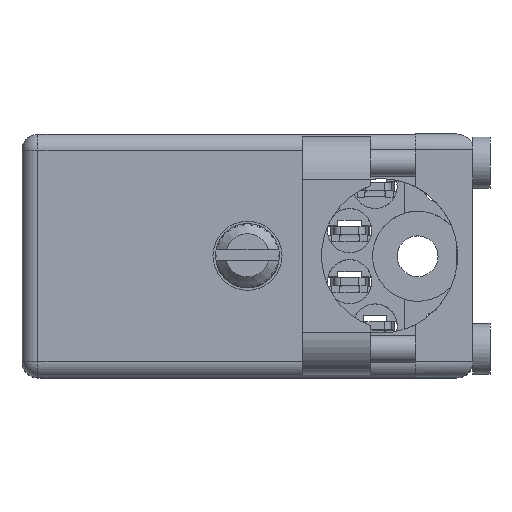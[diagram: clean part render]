
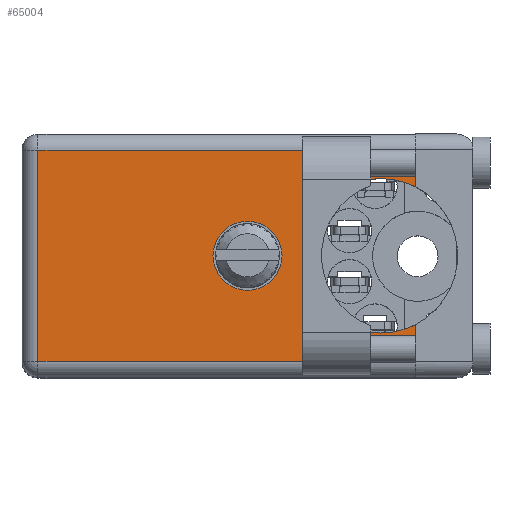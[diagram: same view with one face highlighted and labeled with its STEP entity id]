
A CAD part, top view. The second image highlights one B-rep face of the part: STEP entity #65004.
In plain terms, the highlighted face is planar.
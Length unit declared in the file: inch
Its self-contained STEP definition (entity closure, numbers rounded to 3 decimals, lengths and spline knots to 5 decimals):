
#6867 = AXIS2_PLACEMENT_3D ( 'NONE', #28038, #45267, #128911 ) ;
#7280 = DIRECTION ( 'NONE',  ( -1., 0., 0. ) ) ;
#7720 = CARTESIAN_POINT ( 'NONE',  ( 0.4925, 0.806, -0.3105 ) ) ;
#9717 = EDGE_CURVE ( 'NONE', #14492, #12647, #14792, .T. ) ;
#12647 = VERTEX_POINT ( 'NONE', #168952 ) ;
#12778 = DIRECTION ( 'NONE',  ( 0., 1., 0. ) ) ;
#13889 = AXIS2_PLACEMENT_3D ( 'NONE', #64931, #95680, #7280 ) ;
#14492 = VERTEX_POINT ( 'NONE', #45235 ) ;
#14792 = LINE ( 'NONE', #87786, #27591 ) ;
#18114 = AXIS2_PLACEMENT_3D ( 'NONE', #37521, #50966, #156558 ) ;
#19705 = EDGE_CURVE ( 'NONE', #43490, #105128, #61039, .T. ) ;
#24558 = CIRCLE ( 'NONE', #131970, 0.227 ) ;
#24832 = VERTEX_POINT ( 'NONE', #26908 ) ;
#25369 = ORIENTED_EDGE ( 'NONE', *, *, #111551, .F. ) ;
#26908 = CARTESIAN_POINT ( 'NONE',  ( 0.3905, 0.806, -0.227 ) ) ;
#27200 = CARTESIAN_POINT ( 'NONE',  ( -0.6625, 0.806, -0.3575 ) ) ;
#27327 = CIRCLE ( 'NONE', #18114, 0.227 ) ;
#27591 = VECTOR ( 'NONE', #150162, 39.37008 ) ;
#27747 = LINE ( 'NONE', #142064, #36396 ) ;
#28038 = CARTESIAN_POINT ( 'NONE',  ( 0., 0.806, 0. ) ) ;
#28193 = DIRECTION ( 'NONE',  ( 0., 1., 0. ) ) ;
#31834 = ORIENTED_EDGE ( 'NONE', *, *, #9717, .T. ) ;
#36396 = VECTOR ( 'NONE', #128610, 39.37008 ) ;
#37521 = CARTESIAN_POINT ( 'NONE',  ( 0.3905, 0.806, 0. ) ) ;
#37911 = DIRECTION ( 'NONE',  ( 0., 1., 0. ) ) ;
#40809 = EDGE_CURVE ( 'NONE', #123124, #163807, #27747, .T. ) ;
#41180 = DIRECTION ( 'NONE',  ( 0., 0., 1. ) ) ;
#41448 = CIRCLE ( 'NONE', #13889, 0.227 ) ;
#41816 = ORIENTED_EDGE ( 'NONE', *, *, #19705, .F. ) ;
#43490 = VERTEX_POINT ( 'NONE', #174064 ) ;
#45235 = CARTESIAN_POINT ( 'NONE',  ( -0.6155, 0.806, -0.3105 ) ) ;
#45267 = DIRECTION ( 'NONE',  ( 0., 1., 0. ) ) ;
#46036 = VERTEX_POINT ( 'NONE', #116571 ) ;
#47566 = VERTEX_POINT ( 'NONE', #48930 ) ;
#48930 = CARTESIAN_POINT ( 'NONE',  ( 0.3905, 0.806, 0.227 ) ) ;
#50966 = DIRECTION ( 'NONE',  ( 0., 1., 0. ) ) ;
#52404 = CARTESIAN_POINT ( 'NONE',  ( 0.4925, 0.806, 0.20279 ) ) ;
#59779 = FACE_OUTER_BOUND ( 'NONE', #139218, .T. ) ;
#61039 = CIRCLE ( 'NONE', #6867, 0.1015 ) ;
#64931 = CARTESIAN_POINT ( 'NONE',  ( 0.3905, 0.806, 0. ) ) ;
#65004 = ADVANCED_FACE ( 'NONE', ( #59779, #100188 ), #158760, .T. ) ;
#68299 = EDGE_CURVE ( 'NONE', #24832, #47566, #41448, .T. ) ;
#71351 = DIRECTION ( 'NONE',  ( -1., 0., 0. ) ) ;
#71396 = DIRECTION ( 'NONE',  ( -1., 0., 0. ) ) ;
#74703 = ORIENTED_EDGE ( 'NONE', *, *, #175465, .F. ) ;
#77103 = AXIS2_PLACEMENT_3D ( 'NONE', #27200, #12778, #71351 ) ;
#80381 = CARTESIAN_POINT ( 'NONE',  ( 0.3905, 0.806, 0. ) ) ;
#80827 = LINE ( 'NONE', #123148, #127807 ) ;
#86930 = ORIENTED_EDGE ( 'NONE', *, *, #150568, .T. ) ;
#87745 = AXIS2_PLACEMENT_3D ( 'NONE', #142544, #37911, #100282 ) ;
#87786 = CARTESIAN_POINT ( 'NONE',  ( -0.6155, 0.806, -0.3575 ) ) ;
#89505 = VECTOR ( 'NONE', #162537, 39.37008 ) ;
#90490 = LINE ( 'NONE', #123118, #89505 ) ;
#91344 = EDGE_CURVE ( 'NONE', #105128, #43490, #152193, .T. ) ;
#95680 = DIRECTION ( 'NONE',  ( 0., 1., 0. ) ) ;
#98816 = CARTESIAN_POINT ( 'NONE',  ( 0.4925, 0.806, 0.3575 ) ) ;
#100188 = FACE_BOUND ( 'NONE', #138698, .T. ) ;
#100282 = DIRECTION ( 'NONE',  ( 0., 0., 1. ) ) ;
#103221 = ORIENTED_EDGE ( 'NONE', *, *, #40809, .F. ) ;
#105128 = VERTEX_POINT ( 'NONE', #127263 ) ;
#111551 = EDGE_CURVE ( 'NONE', #189738, #46036, #142991, .T. ) ;
#116571 = CARTESIAN_POINT ( 'NONE',  ( 0.4925, 0.806, 0.3105 ) ) ;
#123118 = CARTESIAN_POINT ( 'NONE',  ( 0.4925, 0.806, 0.3105 ) ) ;
#123124 = VERTEX_POINT ( 'NONE', #7720 ) ;
#123148 = CARTESIAN_POINT ( 'NONE',  ( -0.6625, 0.806, -0.3105 ) ) ;
#125356 = EDGE_CURVE ( 'NONE', #123124, #14492, #80827, .T. ) ;
#127263 = CARTESIAN_POINT ( 'NONE',  ( 0., 0.806, 0.1015 ) ) ;
#127807 = VECTOR ( 'NONE', #139407, 39.37008 ) ;
#128610 = DIRECTION ( 'NONE',  ( 0., 0., 1. ) ) ;
#128911 = DIRECTION ( 'NONE',  ( 0., 0., 1. ) ) ;
#131970 = AXIS2_PLACEMENT_3D ( 'NONE', #80381, #28193, #71396 ) ;
#138698 = EDGE_LOOP ( 'NONE', ( #142811, #41816 ) ) ;
#139218 = EDGE_LOOP ( 'NONE', ( #103221, #141464, #31834, #86930, #25369, #145591, #187707, #74703 ) ) ;
#139407 = DIRECTION ( 'NONE',  ( -1., 0., 0. ) ) ;
#141464 = ORIENTED_EDGE ( 'NONE', *, *, #125356, .T. ) ;
#142064 = CARTESIAN_POINT ( 'NONE',  ( 0.4925, 0.806, 0.3575 ) ) ;
#142544 = CARTESIAN_POINT ( 'NONE',  ( 0., 0.806, 0. ) ) ;
#142811 = ORIENTED_EDGE ( 'NONE', *, *, #91344, .F. ) ;
#142991 = LINE ( 'NONE', #98816, #180203 ) ;
#145591 = ORIENTED_EDGE ( 'NONE', *, *, #180188, .F. ) ;
#150162 = DIRECTION ( 'NONE',  ( 0., 0., 1. ) ) ;
#150568 = EDGE_CURVE ( 'NONE', #12647, #46036, #90490, .T. ) ;
#152193 = CIRCLE ( 'NONE', #87745, 0.1015 ) ;
#156558 = DIRECTION ( 'NONE',  ( -1., 0., 0. ) ) ;
#158760 = PLANE ( 'NONE',  #77103 ) ;
#162537 = DIRECTION ( 'NONE',  ( 1., 0., 0. ) ) ;
#163807 = VERTEX_POINT ( 'NONE', #186714 ) ;
#168952 = CARTESIAN_POINT ( 'NONE',  ( -0.6155, 0.806, 0.3105 ) ) ;
#174064 = CARTESIAN_POINT ( 'NONE',  ( 0., 0.806, -0.1015 ) ) ;
#175465 = EDGE_CURVE ( 'NONE', #163807, #24832, #27327, .T. ) ;
#180188 = EDGE_CURVE ( 'NONE', #47566, #189738, #24558, .T. ) ;
#180203 = VECTOR ( 'NONE', #41180, 39.37008 ) ;
#186714 = CARTESIAN_POINT ( 'NONE',  ( 0.4925, 0.806, -0.20279 ) ) ;
#187707 = ORIENTED_EDGE ( 'NONE', *, *, #68299, .F. ) ;
#189738 = VERTEX_POINT ( 'NONE', #52404 ) ;
